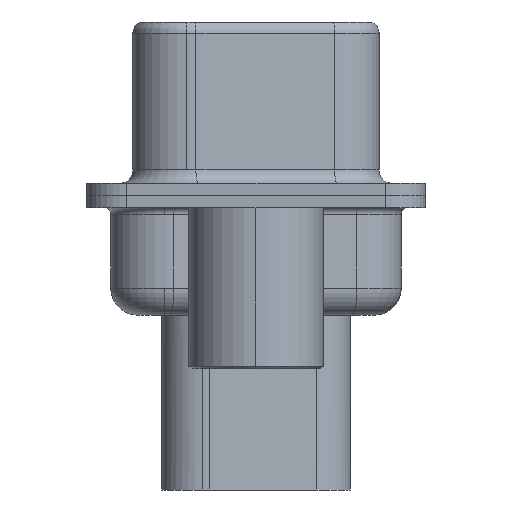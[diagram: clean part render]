
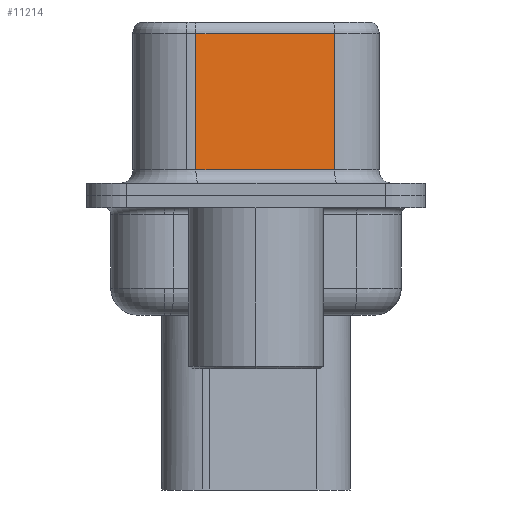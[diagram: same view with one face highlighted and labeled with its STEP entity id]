
A CAD part, left-side view. The second image highlights one B-rep face of the part: STEP entity #11214.
In plain terms, the highlighted planar face has unit normal (-0.985, -0.174, 0).
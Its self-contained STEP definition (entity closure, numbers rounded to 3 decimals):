
#9 = EDGE_LOOP ( 'NONE', ( #12339, #10998, #1609, #15126 ) ) ;
#428 = EDGE_CURVE ( 'NONE', #1940, #8814, #1135, .T. ) ;
#1135 = LINE ( 'NONE', #18617, #14220 ) ;
#1609 = ORIENTED_EDGE ( 'NONE', *, *, #13550, .T. ) ;
#1940 = VERTEX_POINT ( 'NONE', #15088 ) ;
#2201 = VECTOR ( 'NONE', #2513, 1000. ) ;
#2341 = CARTESIAN_POINT ( 'NONE',  ( 4.58, -2.927, 6.02 ) ) ;
#2477 = PLANE ( 'NONE',  #11808 ) ;
#2513 = DIRECTION ( 'NONE',  ( 0., 0., -1. ) ) ;
#4069 = DIRECTION ( 'NONE',  ( 0.985, 0.174, 0. ) ) ;
#5336 = LINE ( 'NONE', #9987, #2201 ) ;
#5845 = VERTEX_POINT ( 'NONE', #15676 ) ;
#6107 = CARTESIAN_POINT ( 'NONE',  ( 4.58, -2.927, 0.95 ) ) ;
#8090 = EDGE_CURVE ( 'NONE', #11974, #8814, #8324, .T. ) ;
#8324 = LINE ( 'NONE', #12697, #12908 ) ;
#8526 = DIRECTION ( 'NONE',  ( 0.174, -0.985, 0. ) ) ;
#8534 = FACE_OUTER_BOUND ( 'NONE', #9, .T. ) ;
#8814 = VERTEX_POINT ( 'NONE', #6107 ) ;
#9073 = DIRECTION ( 'NONE',  ( -0.174, 0.985, 0. ) ) ;
#9722 = EDGE_CURVE ( 'NONE', #11974, #5845, #16313, .T. ) ;
#9987 = CARTESIAN_POINT ( 'NONE',  ( 3.67, 2.233, 6.52 ) ) ;
#10863 = VECTOR ( 'NONE', #9073, 1000. ) ;
#10998 = ORIENTED_EDGE ( 'NONE', *, *, #9722, .T. ) ;
#11214 = ADVANCED_FACE ( 'NONE', ( #8534 ), #2477, .F. ) ;
#11808 = AXIS2_PLACEMENT_3D ( 'NONE', #15869, #4069, #17296 ) ;
#11974 = VERTEX_POINT ( 'NONE', #2341 ) ;
#12339 = ORIENTED_EDGE ( 'NONE', *, *, #8090, .F. ) ;
#12697 = CARTESIAN_POINT ( 'NONE',  ( 4.58, -2.927, 6.52 ) ) ;
#12908 = VECTOR ( 'NONE', #16992, 1000. ) ;
#13466 = CARTESIAN_POINT ( 'NONE',  ( 4.58, -2.927, 6.02 ) ) ;
#13550 = EDGE_CURVE ( 'NONE', #5845, #1940, #5336, .T. ) ;
#14220 = VECTOR ( 'NONE', #8526, 1000. ) ;
#15088 = CARTESIAN_POINT ( 'NONE',  ( 3.67, 2.233, 0.95 ) ) ;
#15126 = ORIENTED_EDGE ( 'NONE', *, *, #428, .T. ) ;
#15676 = CARTESIAN_POINT ( 'NONE',  ( 3.67, 2.233, 6.02 ) ) ;
#15869 = CARTESIAN_POINT ( 'NONE',  ( 4.58, -2.927, 6.52 ) ) ;
#16313 = LINE ( 'NONE', #13466, #10863 ) ;
#16992 = DIRECTION ( 'NONE',  ( 0., 0., -1. ) ) ;
#17296 = DIRECTION ( 'NONE',  ( -0.174, 0.985, 0. ) ) ;
#18617 = CARTESIAN_POINT ( 'NONE',  ( 4.58, -2.927, 0.95 ) ) ;
